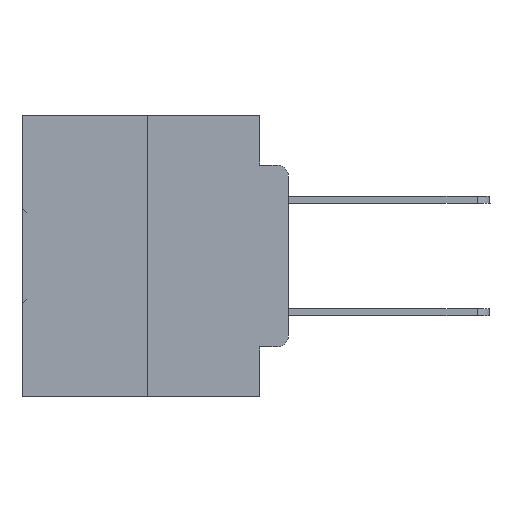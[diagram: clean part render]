
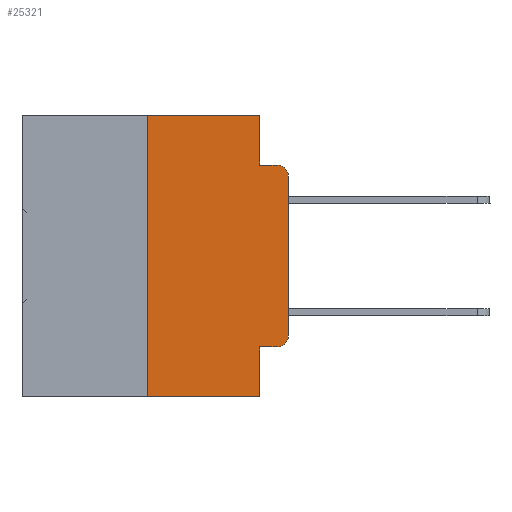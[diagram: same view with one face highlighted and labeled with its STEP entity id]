
A CAD part, left-side view. The second image highlights one B-rep face of the part: STEP entity #25321.
In plain terms, the highlighted planar face has unit normal (-1, 0, 0).
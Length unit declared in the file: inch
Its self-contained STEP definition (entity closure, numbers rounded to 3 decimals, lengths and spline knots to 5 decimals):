
#372 = VERTEX_POINT ( 'NONE', #5689 ) ;
#754 = VERTEX_POINT ( 'NONE', #10528 ) ;
#1611 = CARTESIAN_POINT ( 'NONE',  ( 0., 0.02, -0.1085 ) ) ;
#1963 = EDGE_CURVE ( 'NONE', #5996, #372, #13046, .T. ) ;
#1999 = AXIS2_PLACEMENT_3D ( 'NONE', #32945, #7556, #35290 ) ;
#2260 = DIRECTION ( 'NONE',  ( 0., 0., -1. ) ) ;
#2734 = ORIENTED_EDGE ( 'NONE', *, *, #3497, .F. ) ;
#3497 = EDGE_CURVE ( 'NONE', #9402, #20988, #11810, .T. ) ;
#5189 = VECTOR ( 'NONE', #17819, 39.37008 ) ;
#5689 = CARTESIAN_POINT ( 'NONE',  ( 0., 0., -0.1085 ) ) ;
#5700 = DIRECTION ( 'NONE',  ( 0., 0., 1. ) ) ;
#5996 = VERTEX_POINT ( 'NONE', #22542 ) ;
#6435 = LINE ( 'NONE', #6803, #5189 ) ;
#6803 = CARTESIAN_POINT ( 'NONE',  ( 0., 0.051, 0. ) ) ;
#7556 = DIRECTION ( 'NONE',  ( -1., 0., 0. ) ) ;
#7610 = DIRECTION ( 'NONE',  ( 0., 0., 1. ) ) ;
#9097 = DIRECTION ( 'NONE',  ( 0., 0., -1. ) ) ;
#9402 = VERTEX_POINT ( 'NONE', #32720 ) ;
#9505 = LINE ( 'NONE', #34700, #27768 ) ;
#9691 = CARTESIAN_POINT ( 'NONE',  ( 0., 0.051, -0.0885 ) ) ;
#9836 = DIRECTION ( 'NONE',  ( 0., -1., 0. ) ) ;
#10166 = VERTEX_POINT ( 'NONE', #27343 ) ;
#10265 = DIRECTION ( 'NONE',  ( -1., 0., 0. ) ) ;
#10528 = CARTESIAN_POINT ( 'NONE',  ( 0., 0.051, -0.5 ) ) ;
#11810 = LINE ( 'NONE', #15177, #21531 ) ;
#12281 = EDGE_CURVE ( 'NONE', #22498, #9402, #9505, .T. ) ;
#12283 = EDGE_CURVE ( 'NONE', #21194, #754, #6435, .T. ) ;
#12873 = LINE ( 'NONE', #31777, #27065 ) ;
#12890 = DIRECTION ( 'NONE',  ( 0., -1., 0. ) ) ;
#13046 = LINE ( 'NONE', #24116, #18130 ) ;
#13670 = VECTOR ( 'NONE', #5700, 39.37008 ) ;
#13838 = VECTOR ( 'NONE', #12890, 39.37008 ) ;
#13853 = VERTEX_POINT ( 'NONE', #24369 ) ;
#14584 = ORIENTED_EDGE ( 'NONE', *, *, #12281, .F. ) ;
#14978 = AXIS2_PLACEMENT_3D ( 'NONE', #34697, #32198, #2260 ) ;
#15177 = CARTESIAN_POINT ( 'NONE',  ( 0., 0.051, 0. ) ) ;
#16027 = CARTESIAN_POINT ( 'NONE',  ( 0., 0.25, 0. ) ) ;
#17580 = CIRCLE ( 'NONE', #1999, 0.02 ) ;
#17819 = DIRECTION ( 'NONE',  ( 0., 0., -1. ) ) ;
#18130 = VECTOR ( 'NONE', #7610, 39.37008 ) ;
#18531 = EDGE_CURVE ( 'NONE', #20988, #13853, #20209, .T. ) ;
#19099 = ORIENTED_EDGE ( 'NONE', *, *, #27520, .T. ) ;
#20209 = LINE ( 'NONE', #9691, #34961 ) ;
#20494 = CARTESIAN_POINT ( 'NONE',  ( 0., 0.02, -0.4115 ) ) ;
#20684 = LINE ( 'NONE', #21383, #13838 ) ;
#20988 = VERTEX_POINT ( 'NONE', #26625 ) ;
#21082 = ORIENTED_EDGE ( 'NONE', *, *, #23123, .T. ) ;
#21194 = VERTEX_POINT ( 'NONE', #21871 ) ;
#21383 = CARTESIAN_POINT ( 'NONE',  ( 0., 0.473, -0.5 ) ) ;
#21531 = VECTOR ( 'NONE', #9097, 39.37008 ) ;
#21826 = CARTESIAN_POINT ( 'NONE',  ( 0., 0.25, 0. ) ) ;
#21871 = CARTESIAN_POINT ( 'NONE',  ( 0., 0.051, -0.4115 ) ) ;
#22489 = EDGE_CURVE ( 'NONE', #10166, #22498, #24923, .T. ) ;
#22498 = VERTEX_POINT ( 'NONE', #16027 ) ;
#22542 = CARTESIAN_POINT ( 'NONE',  ( 0., 0., -0.3915 ) ) ;
#23123 = EDGE_CURVE ( 'NONE', #21194, #23174, #12873, .T. ) ;
#23128 = DIRECTION ( 'NONE',  ( 0., -1., 0. ) ) ;
#23174 = VERTEX_POINT ( 'NONE', #20494 ) ;
#23423 = DIRECTION ( 'NONE',  ( 0., -1., 0. ) ) ;
#24116 = CARTESIAN_POINT ( 'NONE',  ( 0., 0., 0. ) ) ;
#24218 = ORIENTED_EDGE ( 'NONE', *, *, #25880, .T. ) ;
#24369 = CARTESIAN_POINT ( 'NONE',  ( 0., 0.02, -0.0885 ) ) ;
#24923 = LINE ( 'NONE', #21826, #13670 ) ;
#25321 = ADVANCED_FACE ( 'NONE', ( #34028 ), #35232, .F. ) ;
#25880 = EDGE_CURVE ( 'NONE', #10166, #754, #20684, .T. ) ;
#26623 = ORIENTED_EDGE ( 'NONE', *, *, #1963, .T. ) ;
#26625 = CARTESIAN_POINT ( 'NONE',  ( 0., 0.051, -0.0885 ) ) ;
#27065 = VECTOR ( 'NONE', #23423, 39.37008 ) ;
#27212 = EDGE_LOOP ( 'NONE', ( #26623, #19099, #28660, #2734, #14584, #27519, #24218, #35699, #21082, #28014 ) ) ;
#27343 = CARTESIAN_POINT ( 'NONE',  ( 0., 0.25, -0.5 ) ) ;
#27519 = ORIENTED_EDGE ( 'NONE', *, *, #22489, .F. ) ;
#27520 = EDGE_CURVE ( 'NONE', #372, #13853, #33667, .T. ) ;
#27768 = VECTOR ( 'NONE', #9836, 39.37008 ) ;
#28014 = ORIENTED_EDGE ( 'NONE', *, *, #32039, .T. ) ;
#28660 = ORIENTED_EDGE ( 'NONE', *, *, #18531, .F. ) ;
#29637 = AXIS2_PLACEMENT_3D ( 'NONE', #1611, #10265, #32083 ) ;
#31777 = CARTESIAN_POINT ( 'NONE',  ( 0., 0.051, -0.4115 ) ) ;
#32039 = EDGE_CURVE ( 'NONE', #23174, #5996, #17580, .T. ) ;
#32083 = DIRECTION ( 'NONE',  ( 0., 0., -1. ) ) ;
#32198 = DIRECTION ( 'NONE',  ( 1., 0., 0. ) ) ;
#32720 = CARTESIAN_POINT ( 'NONE',  ( 0., 0.051, 0. ) ) ;
#32945 = CARTESIAN_POINT ( 'NONE',  ( 0., 0.02, -0.3915 ) ) ;
#33667 = CIRCLE ( 'NONE', #29637, 0.02 ) ;
#34028 = FACE_OUTER_BOUND ( 'NONE', #27212, .T. ) ;
#34697 = CARTESIAN_POINT ( 'NONE',  ( 0., 0.473, 0. ) ) ;
#34700 = CARTESIAN_POINT ( 'NONE',  ( 0., 0.473, 0. ) ) ;
#34961 = VECTOR ( 'NONE', #23128, 39.37008 ) ;
#35232 = PLANE ( 'NONE',  #14978 ) ;
#35290 = DIRECTION ( 'NONE',  ( 0., 0., -1. ) ) ;
#35699 = ORIENTED_EDGE ( 'NONE', *, *, #12283, .F. ) ;
